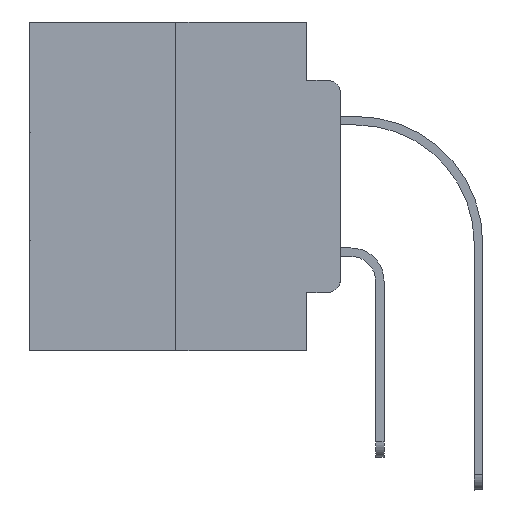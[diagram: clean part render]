
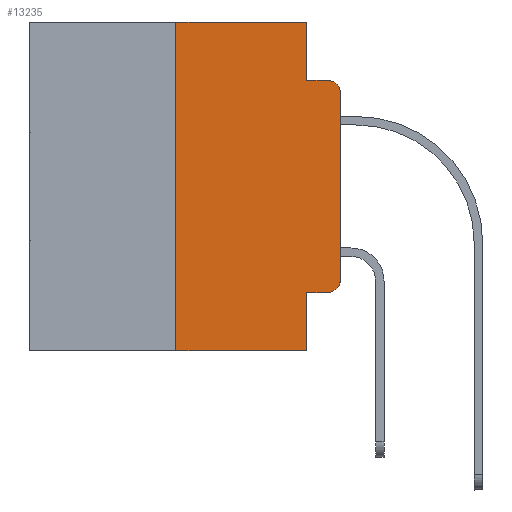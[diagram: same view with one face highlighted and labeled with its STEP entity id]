
A CAD part, left-side view. The second image highlights one B-rep face of the part: STEP entity #13235.
In plain terms, the highlighted planar face has unit normal (-1, 0, 0).
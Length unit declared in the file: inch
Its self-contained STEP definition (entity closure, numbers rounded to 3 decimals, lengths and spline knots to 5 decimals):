
#270 = VERTEX_POINT ( 'NONE', #5281 ) ;
#672 = CARTESIAN_POINT ( 'NONE',  ( 0., 0., -0.3915 ) ) ;
#1465 = AXIS2_PLACEMENT_3D ( 'NONE', #21416, #14575, #3485 ) ;
#2382 = ORIENTED_EDGE ( 'NONE', *, *, #14139, .T. ) ;
#2503 = PLANE ( 'NONE',  #23602 ) ;
#3274 = VERTEX_POINT ( 'NONE', #7022 ) ;
#3485 = DIRECTION ( 'NONE',  ( 0., 0., -1. ) ) ;
#3518 = VERTEX_POINT ( 'NONE', #21535 ) ;
#4097 = CARTESIAN_POINT ( 'NONE',  ( 0., 0.02, -0.0885 ) ) ;
#4297 = VECTOR ( 'NONE', #6969, 39.37008 ) ;
#5182 = DIRECTION ( 'NONE',  ( 0., -1., 0. ) ) ;
#5192 = LINE ( 'NONE', #23117, #4297 ) ;
#5281 = CARTESIAN_POINT ( 'NONE',  ( 0., 0.051, 0. ) ) ;
#5422 = EDGE_CURVE ( 'NONE', #270, #21518, #7191, .T. ) ;
#5604 = ORIENTED_EDGE ( 'NONE', *, *, #20550, .F. ) ;
#5739 = ORIENTED_EDGE ( 'NONE', *, *, #15074, .T. ) ;
#5793 = CARTESIAN_POINT ( 'NONE',  ( 0., 0.25, 0. ) ) ;
#5965 = DIRECTION ( 'NONE',  ( 0., 0., 1. ) ) ;
#6131 = ORIENTED_EDGE ( 'NONE', *, *, #22384, .F. ) ;
#6805 = VERTEX_POINT ( 'NONE', #672 ) ;
#6969 = DIRECTION ( 'NONE',  ( 0., 0., -1. ) ) ;
#7022 = CARTESIAN_POINT ( 'NONE',  ( 0., 0.25, -0.5 ) ) ;
#7190 = DIRECTION ( 'NONE',  ( 0., -1., 0. ) ) ;
#7191 = LINE ( 'NONE', #23188, #27991 ) ;
#7352 = CARTESIAN_POINT ( 'NONE',  ( 0., 0.02, -0.1085 ) ) ;
#7628 = DIRECTION ( 'NONE',  ( 0., 0., 1. ) ) ;
#7694 = CIRCLE ( 'NONE', #22371, 0.02 ) ;
#7706 = ORIENTED_EDGE ( 'NONE', *, *, #23568, .T. ) ;
#8073 = VECTOR ( 'NONE', #7628, 39.37008 ) ;
#8293 = CARTESIAN_POINT ( 'NONE',  ( 0., 0.473, -0.5 ) ) ;
#9195 = LINE ( 'NONE', #11115, #17560 ) ;
#9308 = DIRECTION ( 'NONE',  ( 0., 0., -1. ) ) ;
#9343 = CARTESIAN_POINT ( 'NONE',  ( 0., 0.051, -0.4115 ) ) ;
#9456 = FACE_OUTER_BOUND ( 'NONE', #13849, .T. ) ;
#9583 = CARTESIAN_POINT ( 'NONE',  ( 0., 0., 0. ) ) ;
#9822 = ORIENTED_EDGE ( 'NONE', *, *, #13854, .F. ) ;
#10143 = LINE ( 'NONE', #19182, #15598 ) ;
#10359 = EDGE_CURVE ( 'NONE', #24115, #22727, #7694, .T. ) ;
#10922 = CIRCLE ( 'NONE', #1465, 0.02 ) ;
#11115 = CARTESIAN_POINT ( 'NONE',  ( 0., 0.051, -0.0885 ) ) ;
#11525 = CARTESIAN_POINT ( 'NONE',  ( 0., 0., -0.1085 ) ) ;
#12034 = ORIENTED_EDGE ( 'NONE', *, *, #5422, .F. ) ;
#12982 = ORIENTED_EDGE ( 'NONE', *, *, #24958, .F. ) ;
#13235 = ADVANCED_FACE ( 'NONE', ( #9456 ), #2503, .F. ) ;
#13849 = EDGE_LOOP ( 'NONE', ( #22574, #27822, #6131, #12034, #9822, #12982, #7706, #5604, #2382, #5739 ) ) ;
#13854 = EDGE_CURVE ( 'NONE', #22215, #270, #10143, .T. ) ;
#14139 = EDGE_CURVE ( 'NONE', #24512, #3518, #27126, .T. ) ;
#14548 = CARTESIAN_POINT ( 'NONE',  ( 0., 0.25, 0. ) ) ;
#14575 = DIRECTION ( 'NONE',  ( -1., 0., 0. ) ) ;
#15074 = EDGE_CURVE ( 'NONE', #3518, #6805, #10922, .T. ) ;
#15143 = EDGE_CURVE ( 'NONE', #6805, #24115, #19051, .T. ) ;
#15598 = VECTOR ( 'NONE', #7190, 39.37008 ) ;
#16395 = DIRECTION ( 'NONE',  ( -1., 0., 0. ) ) ;
#16707 = VECTOR ( 'NONE', #17654, 39.37008 ) ;
#17127 = CARTESIAN_POINT ( 'NONE',  ( 0., 0.051, -0.5 ) ) ;
#17560 = VECTOR ( 'NONE', #18078, 39.37008 ) ;
#17654 = DIRECTION ( 'NONE',  ( 0., -1., 0. ) ) ;
#18078 = DIRECTION ( 'NONE',  ( 0., -1., 0. ) ) ;
#18445 = DIRECTION ( 'NONE',  ( 0., 0., -1. ) ) ;
#19051 = LINE ( 'NONE', #9583, #8073 ) ;
#19182 = CARTESIAN_POINT ( 'NONE',  ( 0., 0.473, 0. ) ) ;
#19449 = LINE ( 'NONE', #14548, #22635 ) ;
#20550 = EDGE_CURVE ( 'NONE', #24512, #25988, #5192, .T. ) ;
#20700 = CARTESIAN_POINT ( 'NONE',  ( 0., 0.473, 0. ) ) ;
#21416 = CARTESIAN_POINT ( 'NONE',  ( 0., 0.02, -0.3915 ) ) ;
#21518 = VERTEX_POINT ( 'NONE', #22885 ) ;
#21535 = CARTESIAN_POINT ( 'NONE',  ( 0., 0.02, -0.4115 ) ) ;
#22215 = VERTEX_POINT ( 'NONE', #5793 ) ;
#22371 = AXIS2_PLACEMENT_3D ( 'NONE', #7352, #16395, #25148 ) ;
#22384 = EDGE_CURVE ( 'NONE', #21518, #22727, #9195, .T. ) ;
#22574 = ORIENTED_EDGE ( 'NONE', *, *, #15143, .T. ) ;
#22586 = CARTESIAN_POINT ( 'NONE',  ( 0., 0.051, -0.4115 ) ) ;
#22635 = VECTOR ( 'NONE', #5965, 39.37008 ) ;
#22727 = VERTEX_POINT ( 'NONE', #4097 ) ;
#22885 = CARTESIAN_POINT ( 'NONE',  ( 0., 0.051, -0.0885 ) ) ;
#23117 = CARTESIAN_POINT ( 'NONE',  ( 0., 0.051, 0. ) ) ;
#23188 = CARTESIAN_POINT ( 'NONE',  ( 0., 0.051, 0. ) ) ;
#23189 = VECTOR ( 'NONE', #5182, 39.37008 ) ;
#23568 = EDGE_CURVE ( 'NONE', #3274, #25988, #24325, .T. ) ;
#23602 = AXIS2_PLACEMENT_3D ( 'NONE', #20700, #25161, #9308 ) ;
#24115 = VERTEX_POINT ( 'NONE', #11525 ) ;
#24325 = LINE ( 'NONE', #8293, #16707 ) ;
#24512 = VERTEX_POINT ( 'NONE', #22586 ) ;
#24958 = EDGE_CURVE ( 'NONE', #3274, #22215, #19449, .T. ) ;
#25148 = DIRECTION ( 'NONE',  ( 0., 0., -1. ) ) ;
#25161 = DIRECTION ( 'NONE',  ( 1., 0., 0. ) ) ;
#25988 = VERTEX_POINT ( 'NONE', #17127 ) ;
#27126 = LINE ( 'NONE', #9343, #23189 ) ;
#27822 = ORIENTED_EDGE ( 'NONE', *, *, #10359, .T. ) ;
#27991 = VECTOR ( 'NONE', #18445, 39.37008 ) ;
